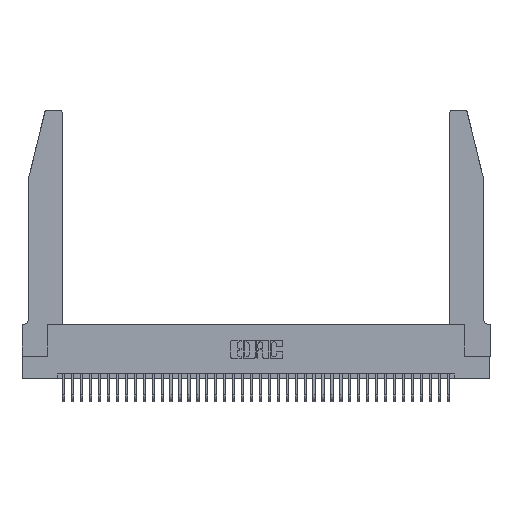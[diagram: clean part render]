
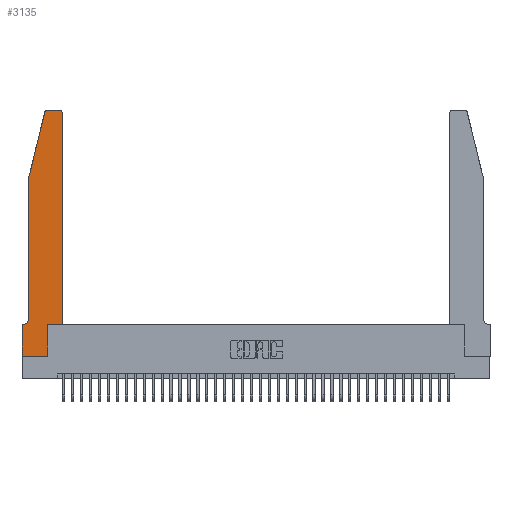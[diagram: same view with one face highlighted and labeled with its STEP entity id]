
A CAD part, top view. The second image highlights one B-rep face of the part: STEP entity #3135.
In plain terms, the highlighted planar face has unit normal (0, 0, 1).
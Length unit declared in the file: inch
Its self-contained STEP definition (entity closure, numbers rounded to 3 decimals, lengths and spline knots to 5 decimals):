
#86 = ORIENTED_EDGE ( 'NONE', *, *, #5131, .T. ) ;
#175 = AXIS2_PLACEMENT_3D ( 'NONE', #38376, #19782, #755 ) ;
#354 = LINE ( 'NONE', #7910, #9940 ) ;
#755 = DIRECTION ( 'NONE',  ( 1., 0., 0. ) ) ;
#830 = VERTEX_POINT ( 'NONE', #18130 ) ;
#1390 = VECTOR ( 'NONE', #38716, 39.37008 ) ;
#1821 = CARTESIAN_POINT ( 'NONE',  ( 0.0755, 0.42, 0.37 ) ) ;
#1891 = CARTESIAN_POINT ( 'NONE',  ( 0.0055, 0.35, 0.37 ) ) ;
#3119 = ORIENTED_EDGE ( 'NONE', *, *, #34462, .T. ) ;
#3135 = ADVANCED_FACE ( 'NONE', ( #25812 ), #32679, .T. ) ;
#3252 = DIRECTION ( 'NONE',  ( 0., 1., 0. ) ) ;
#3320 = DIRECTION ( 'NONE',  ( 0., -1., 0. ) ) ;
#3476 = CARTESIAN_POINT ( 'NONE',  ( 0.284, 2.72, 0.37 ) ) ;
#3996 = LINE ( 'NONE', #29101, #35370 ) ;
#4725 = CARTESIAN_POINT ( 'NONE',  ( 0.4505, 0.35, 0.37 ) ) ;
#5020 = CARTESIAN_POINT ( 'NONE',  ( 0.0055, 0.42, 0.37 ) ) ;
#5131 = EDGE_CURVE ( 'NONE', #830, #9483, #28760, .T. ) ;
#5143 = VERTEX_POINT ( 'NONE', #35271 ) ;
#5270 = EDGE_LOOP ( 'NONE', ( #35337, #27063, #32732, #36220, #33968, #3119, #23374, #17800, #37606, #33773, #9287, #86 ) ) ;
#5316 = VERTEX_POINT ( 'NONE', #11319 ) ;
#6058 = VERTEX_POINT ( 'NONE', #18380 ) ;
#6725 = DIRECTION ( 'NONE',  ( 1., 0., 0. ) ) ;
#7846 = DIRECTION ( 'NONE',  ( 1., 0., 0. ) ) ;
#7910 = CARTESIAN_POINT ( 'NONE',  ( 0., 0., 0.37 ) ) ;
#7932 = DIRECTION ( 'NONE',  ( 1., 0., 0. ) ) ;
#8206 = DIRECTION ( 'NONE',  ( -1., 0., 0. ) ) ;
#9287 = ORIENTED_EDGE ( 'NONE', *, *, #12039, .T. ) ;
#9483 = VERTEX_POINT ( 'NONE', #13597 ) ;
#9940 = VECTOR ( 'NONE', #29733, 39.37008 ) ;
#10106 = CARTESIAN_POINT ( 'NONE',  ( 0.4505, 0.35, 0.37 ) ) ;
#10477 = CARTESIAN_POINT ( 'NONE',  ( 0., 0.35, 0.37 ) ) ;
#10573 = EDGE_CURVE ( 'NONE', #5143, #29729, #20593, .T. ) ;
#11104 = CARTESIAN_POINT ( 'NONE',  ( 0.0755, 0.35, 0.37 ) ) ;
#11319 = CARTESIAN_POINT ( 'NONE',  ( 0., 0., 0.37 ) ) ;
#12039 = EDGE_CURVE ( 'NONE', #19500, #830, #14538, .T. ) ;
#13027 = EDGE_CURVE ( 'NONE', #39115, #32447, #3996, .T. ) ;
#13597 = CARTESIAN_POINT ( 'NONE',  ( 0.4205, 2.75, 0.37 ) ) ;
#13774 = EDGE_CURVE ( 'NONE', #29729, #39115, #26515, .T. ) ;
#13814 = EDGE_CURVE ( 'NONE', #5316, #31048, #354, .T. ) ;
#14153 = AXIS2_PLACEMENT_3D ( 'NONE', #3476, #25473, #6725 ) ;
#14538 = LINE ( 'NONE', #10106, #30080 ) ;
#15925 = CARTESIAN_POINT ( 'NONE',  ( 0.2865, 0.35, 0.37 ) ) ;
#16512 = CARTESIAN_POINT ( 'NONE',  ( 0.0755, 2., 0.37 ) ) ;
#16542 = VECTOR ( 'NONE', #3320, 39.37008 ) ;
#16917 = CIRCLE ( 'NONE', #18852, 0.07 ) ;
#16962 = LINE ( 'NONE', #24175, #32509 ) ;
#17586 = VECTOR ( 'NONE', #3252, 39.37008 ) ;
#17800 = ORIENTED_EDGE ( 'NONE', *, *, #13814, .T. ) ;
#18062 = DIRECTION ( 'NONE',  ( -1., 0., 0. ) ) ;
#18130 = CARTESIAN_POINT ( 'NONE',  ( 0.4505, 2.72, 0.37 ) ) ;
#18380 = CARTESIAN_POINT ( 'NONE',  ( 0.2865, 0.35, 0.37 ) ) ;
#18852 = AXIS2_PLACEMENT_3D ( 'NONE', #5020, #26883, #8206 ) ;
#19261 = CARTESIAN_POINT ( 'NONE',  ( 0.4505, 0.35, 0.37 ) ) ;
#19500 = VERTEX_POINT ( 'NONE', #19261 ) ;
#19782 = DIRECTION ( 'NONE',  ( 0., 0., 1. ) ) ;
#19946 = CARTESIAN_POINT ( 'NONE',  ( 0.2865, 0., 0.37 ) ) ;
#20258 = CARTESIAN_POINT ( 'NONE',  ( 0.0755, 2., 0.37 ) ) ;
#20514 = DIRECTION ( 'NONE',  ( -1., 0., 0. ) ) ;
#20593 = CIRCLE ( 'NONE', #14153, 0.03 ) ;
#20814 = EDGE_CURVE ( 'NONE', #31048, #6058, #25836, .T. ) ;
#21247 = VECTOR ( 'NONE', #20514, 39.37008 ) ;
#21728 = LINE ( 'NONE', #4725, #37291 ) ;
#22881 = DIRECTION ( 'NONE',  ( 0., -1., 0. ) ) ;
#23374 = ORIENTED_EDGE ( 'NONE', *, *, #39019, .T. ) ;
#23455 = CARTESIAN_POINT ( 'NONE',  ( 0., 0.35, 0.37 ) ) ;
#23744 = EDGE_CURVE ( 'NONE', #6058, #19500, #21728, .T. ) ;
#24175 = CARTESIAN_POINT ( 'NONE',  ( 0.2605, 2.75, 0.37 ) ) ;
#25322 = CARTESIAN_POINT ( 'NONE',  ( 0., 0., 0.37 ) ) ;
#25473 = DIRECTION ( 'NONE',  ( 0., 0., 1. ) ) ;
#25812 = FACE_OUTER_BOUND ( 'NONE', #5270, .T. ) ;
#25836 = LINE ( 'NONE', #15925, #17586 ) ;
#26515 = LINE ( 'NONE', #20258, #1390 ) ;
#26529 = DIRECTION ( 'NONE',  ( 0., 0., 1. ) ) ;
#26883 = DIRECTION ( 'NONE',  ( 0., 0., -1. ) ) ;
#27063 = ORIENTED_EDGE ( 'NONE', *, *, #10573, .T. ) ;
#28521 = EDGE_CURVE ( 'NONE', #9483, #5143, #16962, .T. ) ;
#28760 = CIRCLE ( 'NONE', #175, 0.03 ) ;
#29101 = CARTESIAN_POINT ( 'NONE',  ( 0.0755, 2., 0.37 ) ) ;
#29483 = LINE ( 'NONE', #11104, #21247 ) ;
#29729 = VERTEX_POINT ( 'NONE', #38357 ) ;
#29733 = DIRECTION ( 'NONE',  ( 1., 0., 0. ) ) ;
#30080 = VECTOR ( 'NONE', #38159, 39.37008 ) ;
#30244 = AXIS2_PLACEMENT_3D ( 'NONE', #23455, #26529, #7846 ) ;
#31048 = VERTEX_POINT ( 'NONE', #19946 ) ;
#32076 = LINE ( 'NONE', #25322, #16542 ) ;
#32447 = VERTEX_POINT ( 'NONE', #1821 ) ;
#32509 = VECTOR ( 'NONE', #18062, 39.37008 ) ;
#32679 = PLANE ( 'NONE',  #30244 ) ;
#32732 = ORIENTED_EDGE ( 'NONE', *, *, #13774, .T. ) ;
#33773 = ORIENTED_EDGE ( 'NONE', *, *, #23744, .T. ) ;
#33888 = EDGE_CURVE ( 'NONE', #32447, #39394, #16917, .T. ) ;
#33968 = ORIENTED_EDGE ( 'NONE', *, *, #33888, .T. ) ;
#34462 = EDGE_CURVE ( 'NONE', #39394, #35887, #29483, .T. ) ;
#35271 = CARTESIAN_POINT ( 'NONE',  ( 0.284, 2.75, 0.37 ) ) ;
#35337 = ORIENTED_EDGE ( 'NONE', *, *, #28521, .T. ) ;
#35370 = VECTOR ( 'NONE', #22881, 39.37008 ) ;
#35887 = VERTEX_POINT ( 'NONE', #10477 ) ;
#36220 = ORIENTED_EDGE ( 'NONE', *, *, #13027, .T. ) ;
#37291 = VECTOR ( 'NONE', #7932, 39.37008 ) ;
#37606 = ORIENTED_EDGE ( 'NONE', *, *, #20814, .T. ) ;
#38159 = DIRECTION ( 'NONE',  ( 0., 1., 0. ) ) ;
#38357 = CARTESIAN_POINT ( 'NONE',  ( 0.25487, 2.72718, 0.37 ) ) ;
#38376 = CARTESIAN_POINT ( 'NONE',  ( 0.4205, 2.72, 0.37 ) ) ;
#38716 = DIRECTION ( 'NONE',  ( -0.239, -0.971, 0. ) ) ;
#39019 = EDGE_CURVE ( 'NONE', #35887, #5316, #32076, .T. ) ;
#39115 = VERTEX_POINT ( 'NONE', #16512 ) ;
#39394 = VERTEX_POINT ( 'NONE', #1891 ) ;
